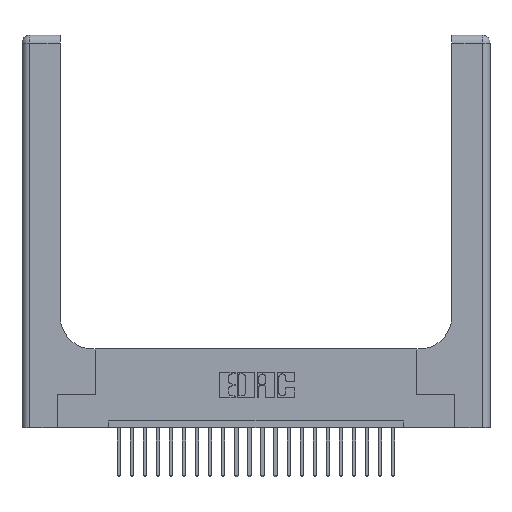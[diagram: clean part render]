
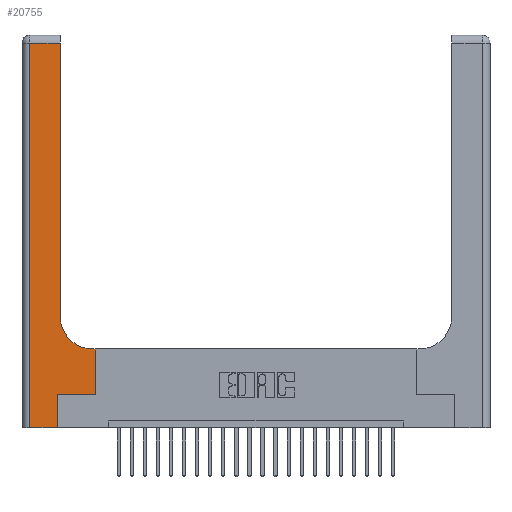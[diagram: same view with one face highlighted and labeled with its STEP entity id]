
A CAD part, top view. The second image highlights one B-rep face of the part: STEP entity #20755.
In plain terms, the highlighted planar face has unit normal (0, 0, 1).
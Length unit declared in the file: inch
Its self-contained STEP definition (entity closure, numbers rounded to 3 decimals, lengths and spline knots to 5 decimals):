
#23 = DIRECTION ( 'NONE',  ( 0., 1., 0. ) ) ;
#220 = CARTESIAN_POINT ( 'NONE',  ( 0.269, 0., 0.37 ) ) ;
#1636 = CARTESIAN_POINT ( 'NONE',  ( 0.5415, 0.6, 0.37 ) ) ;
#2105 = EDGE_CURVE ( 'NONE', #10274, #22521, #17865, .T. ) ;
#2177 = VERTEX_POINT ( 'NONE', #24352 ) ;
#2207 = DIRECTION ( 'NONE',  ( 0., -1., 0. ) ) ;
#2525 = EDGE_LOOP ( 'NONE', ( #12798, #15334, #14453, #8076, #21831, #12265, #12172, #3745, #10243 ) ) ;
#3151 = VERTEX_POINT ( 'NONE', #16708 ) ;
#3732 = AXIS2_PLACEMENT_3D ( 'NONE', #18154, #17885, #17979 ) ;
#3745 = ORIENTED_EDGE ( 'NONE', *, *, #12491, .T. ) ;
#3941 = CARTESIAN_POINT ( 'NONE',  ( 0.06, 3., 0.37 ) ) ;
#3977 = VECTOR ( 'NONE', #4293, 39.37008 ) ;
#4293 = DIRECTION ( 'NONE',  ( 1., 0., 0. ) ) ;
#5296 = CARTESIAN_POINT ( 'NONE',  ( 0.269, 0., 0.37 ) ) ;
#5487 = AXIS2_PLACEMENT_3D ( 'NONE', #15432, #17609, #17352 ) ;
#5550 = CARTESIAN_POINT ( 'NONE',  ( 0.5585, 0.25, 0.37 ) ) ;
#6210 = DIRECTION ( 'NONE',  ( -1., 0., 0. ) ) ;
#6448 = CARTESIAN_POINT ( 'NONE',  ( 0., 0., 0.37 ) ) ;
#8076 = ORIENTED_EDGE ( 'NONE', *, *, #17837, .T. ) ;
#8170 = VERTEX_POINT ( 'NONE', #20601 ) ;
#8694 = LINE ( 'NONE', #6448, #3977 ) ;
#9053 = EDGE_CURVE ( 'NONE', #22887, #9701, #11668, .T. ) ;
#9701 = VERTEX_POINT ( 'NONE', #12548 ) ;
#9784 = LINE ( 'NONE', #19582, #19576 ) ;
#10243 = ORIENTED_EDGE ( 'NONE', *, *, #9053, .T. ) ;
#10274 = VERTEX_POINT ( 'NONE', #220 ) ;
#10333 = VERTEX_POINT ( 'NONE', #23428 ) ;
#11053 = EDGE_CURVE ( 'NONE', #3151, #2177, #20221, .T. ) ;
#11668 = CIRCLE ( 'NONE', #5487, 0.25 ) ;
#12172 = ORIENTED_EDGE ( 'NONE', *, *, #11053, .T. ) ;
#12191 = CARTESIAN_POINT ( 'NONE',  ( 0.06, 2.94, 0.37 ) ) ;
#12265 = ORIENTED_EDGE ( 'NONE', *, *, #12511, .T. ) ;
#12491 = EDGE_CURVE ( 'NONE', #2177, #22887, #16609, .T. ) ;
#12511 = EDGE_CURVE ( 'NONE', #22521, #3151, #9784, .T. ) ;
#12548 = CARTESIAN_POINT ( 'NONE',  ( 0.2915, 0.85, 0.37 ) ) ;
#12584 = FACE_OUTER_BOUND ( 'NONE', #2525, .T. ) ;
#12798 = ORIENTED_EDGE ( 'NONE', *, *, #16764, .T. ) ;
#13776 = CARTESIAN_POINT ( 'NONE',  ( 0.2915, 0.6, 0.37 ) ) ;
#14070 = LINE ( 'NONE', #3941, #20874 ) ;
#14453 = ORIENTED_EDGE ( 'NONE', *, *, #20567, .T. ) ;
#14623 = DIRECTION ( 'NONE',  ( 0., 1., 0. ) ) ;
#14875 = VECTOR ( 'NONE', #14623, 39.37008 ) ;
#15020 = VECTOR ( 'NONE', #15876, 39.37008 ) ;
#15334 = ORIENTED_EDGE ( 'NONE', *, *, #18858, .T. ) ;
#15432 = CARTESIAN_POINT ( 'NONE',  ( 0.5415, 0.85, 0.37 ) ) ;
#15599 = DIRECTION ( 'NONE',  ( 1., 0., 0. ) ) ;
#15876 = DIRECTION ( 'NONE',  ( -1., 0., 0. ) ) ;
#15985 = DIRECTION ( 'NONE',  ( 0., 1., 0. ) ) ;
#16066 = VECTOR ( 'NONE', #23, 39.37008 ) ;
#16209 = PLANE ( 'NONE',  #3732 ) ;
#16609 = LINE ( 'NONE', #13776, #24282 ) ;
#16708 = CARTESIAN_POINT ( 'NONE',  ( 0.5585, 0.25, 0.37 ) ) ;
#16764 = EDGE_CURVE ( 'NONE', #9701, #10333, #19682, .T. ) ;
#17352 = DIRECTION ( 'NONE',  ( 1., 0., 0. ) ) ;
#17609 = DIRECTION ( 'NONE',  ( 0., 0., -1. ) ) ;
#17837 = EDGE_CURVE ( 'NONE', #8170, #10274, #8694, .T. ) ;
#17865 = LINE ( 'NONE', #5296, #14875 ) ;
#17885 = DIRECTION ( 'NONE',  ( 0., 0., -1. ) ) ;
#17964 = CARTESIAN_POINT ( 'NONE',  ( 0., 2.94, 0.37 ) ) ;
#17979 = DIRECTION ( 'NONE',  ( -1., 0., 0. ) ) ;
#18154 = CARTESIAN_POINT ( 'NONE',  ( 0., 3., 0.37 ) ) ;
#18858 = EDGE_CURVE ( 'NONE', #10333, #22588, #20072, .T. ) ;
#19250 = CARTESIAN_POINT ( 'NONE',  ( 0.269, 0.25, 0.37 ) ) ;
#19576 = VECTOR ( 'NONE', #15599, 39.37008 ) ;
#19582 = CARTESIAN_POINT ( 'NONE',  ( 0.269, 0.25, 0.37 ) ) ;
#19682 = LINE ( 'NONE', #21545, #24396 ) ;
#20072 = LINE ( 'NONE', #17964, #15020 ) ;
#20221 = LINE ( 'NONE', #5550, #16066 ) ;
#20567 = EDGE_CURVE ( 'NONE', #22588, #8170, #14070, .T. ) ;
#20601 = CARTESIAN_POINT ( 'NONE',  ( 0.06, 0., 0.37 ) ) ;
#20755 = ADVANCED_FACE ( 'NONE', ( #12584 ), #16209, .F. ) ;
#20874 = VECTOR ( 'NONE', #2207, 39.37008 ) ;
#21545 = CARTESIAN_POINT ( 'NONE',  ( 0.2915, 3., 0.37 ) ) ;
#21831 = ORIENTED_EDGE ( 'NONE', *, *, #2105, .T. ) ;
#22521 = VERTEX_POINT ( 'NONE', #19250 ) ;
#22588 = VERTEX_POINT ( 'NONE', #12191 ) ;
#22887 = VERTEX_POINT ( 'NONE', #1636 ) ;
#23428 = CARTESIAN_POINT ( 'NONE',  ( 0.2915, 2.94, 0.37 ) ) ;
#24282 = VECTOR ( 'NONE', #6210, 39.37008 ) ;
#24352 = CARTESIAN_POINT ( 'NONE',  ( 0.5585, 0.6, 0.37 ) ) ;
#24396 = VECTOR ( 'NONE', #15985, 39.37008 ) ;
